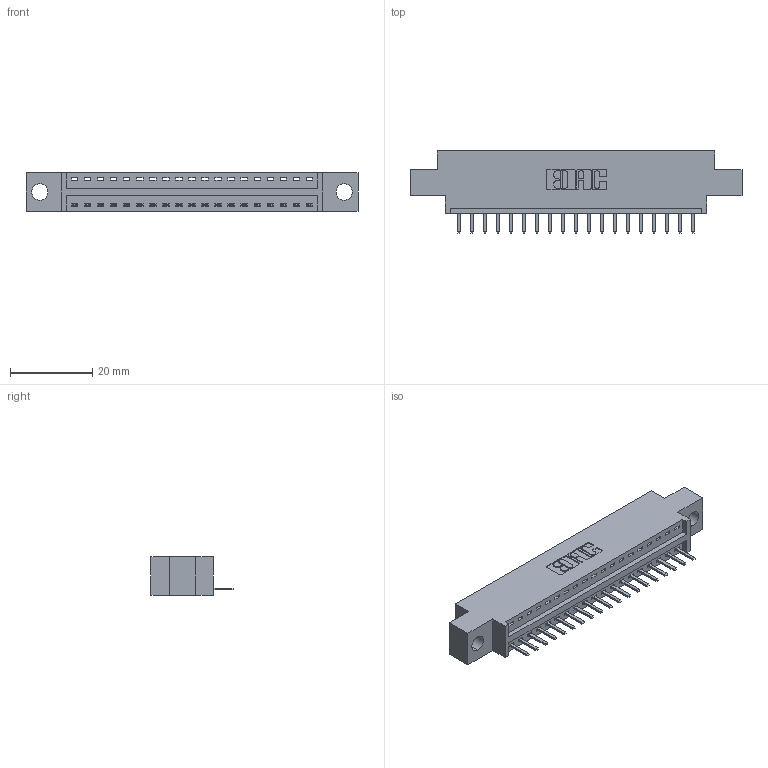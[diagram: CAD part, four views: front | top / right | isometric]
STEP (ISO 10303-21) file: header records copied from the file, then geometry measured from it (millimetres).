
FILE_DESCRIPTION (( 'STEP AP203' ), '1' );
FILE_NAME ('346-019-520-604.STEP', '2022-05-05T15:00:17', ( '' ), ( '' ), 'SwSTEP 2.0', 'SolidWorks 2020', '' );
FILE_SCHEMA (( 'CONFIG_CONTROL_DESIGN' ));
Length unit declared in the file: inch
Products named in the file (3): 345-292-001_345-293-120; 346-019-520-604; 346 Part_0.170 Offset - 0.156 Dia-TH
Assembly tree (20 placements, depth 2):
  346-019-520-604
    346 Part_0.170 Offset - 0.156 Dia-TH
    345-292-001_345-293-120  x19
Bounding box: 80.9 x 20.02 x 9.4 mm (x, y, z)
Volume: 7270.1 mm3; surface area: 8653.7 mm2
Topology: 20 solids, 20 shells, 1318 faces, 3873 edges, 2530 vertices
Faces by surface type: plane 892, cylinder 426
Entity records: 15553 total; most frequent: CARTESIAN_POINT 2695, ORIENTED_EDGE 2634, DIRECTION 2391, EDGE_CURVE 1317, VECTOR 1105, LINE 1105, VERTEX_POINT 874, AXIS2_PLACEMENT_3D 643
